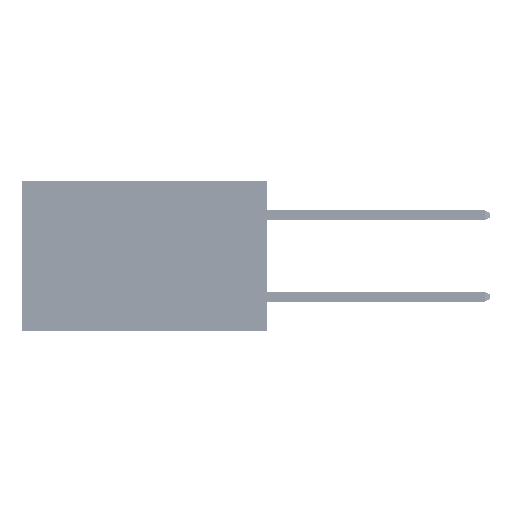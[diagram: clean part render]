
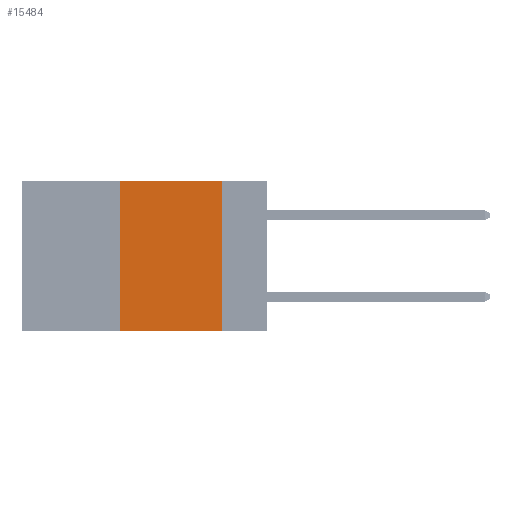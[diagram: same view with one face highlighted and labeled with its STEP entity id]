
A CAD part, left-side view. The second image highlights one B-rep face of the part: STEP entity #15484.
In plain terms, the highlighted planar face has unit normal (-1, 0, 0).
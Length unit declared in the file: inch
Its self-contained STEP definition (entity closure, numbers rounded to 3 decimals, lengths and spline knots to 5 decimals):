
#468 = DIRECTION ( 'NONE',  ( 0., 0., -1. ) ) ;
#1949 = LINE ( 'NONE', #23220, #43419 ) ;
#4153 = FACE_OUTER_BOUND ( 'NONE', #12598, .T. ) ;
#8362 = VERTEX_POINT ( 'NONE', #51814 ) ;
#12483 = CARTESIAN_POINT ( 'NONE',  ( 0., 0.36, 0. ) ) ;
#12598 = EDGE_LOOP ( 'NONE', ( #25182, #23774, #24605, #20081 ) ) ;
#15252 = VECTOR ( 'NONE', #51372, 39.37008 ) ;
#15484 = ADVANCED_FACE ( 'NONE', ( #4153 ), #20536, .F. ) ;
#16520 = CARTESIAN_POINT ( 'NONE',  ( 0., 0.6, 0. ) ) ;
#16883 = CARTESIAN_POINT ( 'NONE',  ( 0., 0.11, 0. ) ) ;
#19016 = EDGE_CURVE ( 'NONE', #8362, #31808, #1949, .T. ) ;
#19310 = CARTESIAN_POINT ( 'NONE',  ( 0., 0.6, 0. ) ) ;
#19895 = VERTEX_POINT ( 'NONE', #48030 ) ;
#20081 = ORIENTED_EDGE ( 'NONE', *, *, #19016, .T. ) ;
#20191 = VERTEX_POINT ( 'NONE', #33646 ) ;
#20536 = PLANE ( 'NONE',  #37071 ) ;
#20945 = LINE ( 'NONE', #12483, #49156 ) ;
#23220 = CARTESIAN_POINT ( 'NONE',  ( 0., 0.6, -0.37 ) ) ;
#23774 = ORIENTED_EDGE ( 'NONE', *, *, #51966, .F. ) ;
#24582 = DIRECTION ( 'NONE',  ( 1., 0., 0. ) ) ;
#24605 = ORIENTED_EDGE ( 'NONE', *, *, #34260, .F. ) ;
#25182 = ORIENTED_EDGE ( 'NONE', *, *, #32516, .F. ) ;
#26806 = VECTOR ( 'NONE', #33027, 39.37008 ) ;
#28720 = CARTESIAN_POINT ( 'NONE',  ( 0., 0.11, -0.37 ) ) ;
#31808 = VERTEX_POINT ( 'NONE', #28720 ) ;
#32516 = EDGE_CURVE ( 'NONE', #19895, #31808, #37483, .T. ) ;
#33027 = DIRECTION ( 'NONE',  ( 0., 0., -1. ) ) ;
#33646 = CARTESIAN_POINT ( 'NONE',  ( 0., 0.36, 0. ) ) ;
#34260 = EDGE_CURVE ( 'NONE', #8362, #20191, #20945, .T. ) ;
#36503 = DIRECTION ( 'NONE',  ( 0., 0., 1. ) ) ;
#37071 = AXIS2_PLACEMENT_3D ( 'NONE', #16520, #24582, #468 ) ;
#37483 = LINE ( 'NONE', #16883, #26806 ) ;
#37860 = LINE ( 'NONE', #19310, #15252 ) ;
#43419 = VECTOR ( 'NONE', #51247, 39.37008 ) ;
#48030 = CARTESIAN_POINT ( 'NONE',  ( 0., 0.11, 0. ) ) ;
#49156 = VECTOR ( 'NONE', #36503, 39.37008 ) ;
#51247 = DIRECTION ( 'NONE',  ( 0., -1., 0. ) ) ;
#51372 = DIRECTION ( 'NONE',  ( 0., -1., 0. ) ) ;
#51814 = CARTESIAN_POINT ( 'NONE',  ( 0., 0.36, -0.37 ) ) ;
#51966 = EDGE_CURVE ( 'NONE', #20191, #19895, #37860, .T. ) ;
